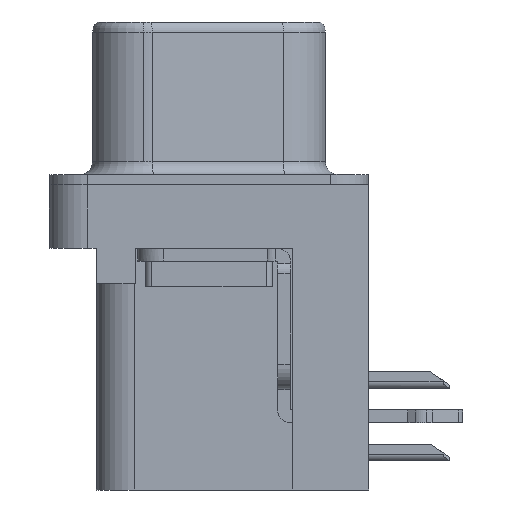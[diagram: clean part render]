
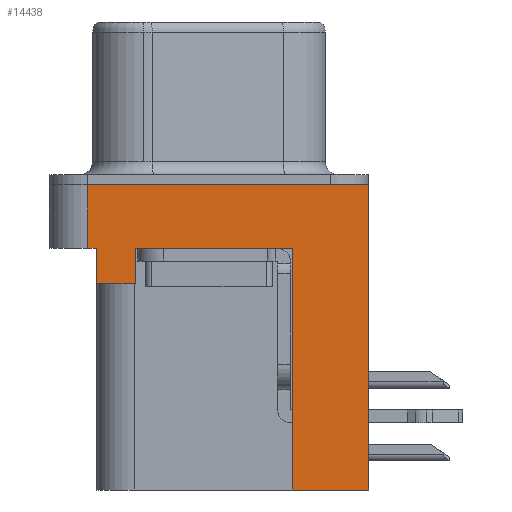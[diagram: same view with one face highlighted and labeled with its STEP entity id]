
A CAD part, left-side view. The second image highlights one B-rep face of the part: STEP entity #14438.
In plain terms, the highlighted planar face has unit normal (-1, 0, 0).
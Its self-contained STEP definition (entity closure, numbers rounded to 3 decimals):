
#424 = CARTESIAN_POINT ( 'NONE',  ( -2.91, -3.295, -12. ) ) ;
#498 = LINE ( 'NONE', #3446, #7345 ) ;
#590 = CARTESIAN_POINT ( 'NONE',  ( -2.91, -6.275, -12. ) ) ;
#839 = LINE ( 'NONE', #424, #10477 ) ;
#1128 = ORIENTED_EDGE ( 'NONE', *, *, #12893, .T. ) ;
#1135 = EDGE_CURVE ( 'NONE', #9206, #2149, #12615, .T. ) ;
#1337 = CARTESIAN_POINT ( 'NONE',  ( -2.91, -6.275, -2.5 ) ) ;
#1346 = CARTESIAN_POINT ( 'NONE',  ( -2.91, -6.275, -2.5 ) ) ;
#1500 = DIRECTION ( 'NONE',  ( 0., 1., 0. ) ) ;
#1649 = VECTOR ( 'NONE', #1500, 1000. ) ;
#1783 = VERTEX_POINT ( 'NONE', #590 ) ;
#1950 = VERTEX_POINT ( 'NONE', #9970 ) ;
#1992 = ORIENTED_EDGE ( 'NONE', *, *, #14598, .F. ) ;
#2149 = VERTEX_POINT ( 'NONE', #2398 ) ;
#2398 = CARTESIAN_POINT ( 'NONE',  ( -2.91, 4.425, -2.5 ) ) ;
#2437 = ORIENTED_EDGE ( 'NONE', *, *, #13049, .F. ) ;
#2489 = CARTESIAN_POINT ( 'NONE',  ( -2.91, 4.775, -2.5 ) ) ;
#2732 = CARTESIAN_POINT ( 'NONE',  ( -2.91, 2.895, -3.9 ) ) ;
#2968 = CARTESIAN_POINT ( 'NONE',  ( -2.91, 2.895, -3.9 ) ) ;
#3211 = CARTESIAN_POINT ( 'NONE',  ( -2.91, -6.275, 0. ) ) ;
#3323 = CARTESIAN_POINT ( 'NONE',  ( -2.91, 4.425, -3.9 ) ) ;
#3330 = DIRECTION ( 'NONE',  ( 0., -1., 0. ) ) ;
#3446 = CARTESIAN_POINT ( 'NONE',  ( -2.91, 4.425, -3.9 ) ) ;
#3449 = FACE_OUTER_BOUND ( 'NONE', #11351, .T. ) ;
#3548 = CARTESIAN_POINT ( 'NONE',  ( -2.91, 4.425, -3.9 ) ) ;
#3819 = EDGE_CURVE ( 'NONE', #14897, #7387, #4460, .T. ) ;
#4460 = LINE ( 'NONE', #3211, #14893 ) ;
#4625 = LINE ( 'NONE', #5019, #14853 ) ;
#5019 = CARTESIAN_POINT ( 'NONE',  ( -2.91, 4.775, -2.5 ) ) ;
#5184 = ORIENTED_EDGE ( 'NONE', *, *, #1135, .T. ) ;
#5431 = CARTESIAN_POINT ( 'NONE',  ( -2.91, -3.295, -12. ) ) ;
#5680 = CARTESIAN_POINT ( 'NONE',  ( -2.91, -6.275, -2.5 ) ) ;
#5758 = ORIENTED_EDGE ( 'NONE', *, *, #7703, .F. ) ;
#6206 = DIRECTION ( 'NONE',  ( 0., 1., 0. ) ) ;
#6289 = DIRECTION ( 'NONE',  ( 0., 0., 1. ) ) ;
#7345 = VECTOR ( 'NONE', #9887, 1000. ) ;
#7378 = DIRECTION ( 'NONE',  ( 0., 0., 1. ) ) ;
#7387 = VERTEX_POINT ( 'NONE', #10340 ) ;
#7674 = LINE ( 'NONE', #5431, #1649 ) ;
#7703 = EDGE_CURVE ( 'NONE', #15820, #10957, #13242, .T. ) ;
#8428 = ORIENTED_EDGE ( 'NONE', *, *, #13029, .F. ) ;
#8457 = VECTOR ( 'NONE', #10475, 1000. ) ;
#8480 = CARTESIAN_POINT ( 'NONE',  ( -2.91, -6.275, -2.5 ) ) ;
#8582 = VERTEX_POINT ( 'NONE', #11330 ) ;
#8858 = LINE ( 'NONE', #2968, #8457 ) ;
#9206 = VERTEX_POINT ( 'NONE', #2489 ) ;
#9887 = DIRECTION ( 'NONE',  ( 0., 0., 1. ) ) ;
#9970 = CARTESIAN_POINT ( 'NONE',  ( -2.91, 2.895, -2.5 ) ) ;
#10340 = CARTESIAN_POINT ( 'NONE',  ( -2.91, -6.275, 0. ) ) ;
#10442 = EDGE_CURVE ( 'NONE', #1950, #14710, #11135, .T. ) ;
#10475 = DIRECTION ( 'NONE',  ( 0., 0., 1. ) ) ;
#10477 = VECTOR ( 'NONE', #11759, 1000. ) ;
#10670 = LINE ( 'NONE', #1337, #11669 ) ;
#10957 = VERTEX_POINT ( 'NONE', #3323 ) ;
#10972 = EDGE_CURVE ( 'NONE', #10957, #2149, #498, .T. ) ;
#11135 = LINE ( 'NONE', #1346, #12361 ) ;
#11266 = CARTESIAN_POINT ( 'NONE',  ( -2.91, 4.775, 0. ) ) ;
#11330 = CARTESIAN_POINT ( 'NONE',  ( -2.91, -3.295, -12. ) ) ;
#11351 = EDGE_LOOP ( 'NONE', ( #13111, #1992, #5184, #11954, #5758, #15633, #11935, #2437, #8428, #1128 ) ) ;
#11669 = VECTOR ( 'NONE', #14252, 1000. ) ;
#11759 = DIRECTION ( 'NONE',  ( 0., 0., 1. ) ) ;
#11935 = ORIENTED_EDGE ( 'NONE', *, *, #10442, .T. ) ;
#11954 = ORIENTED_EDGE ( 'NONE', *, *, #10972, .F. ) ;
#12237 = VECTOR ( 'NONE', #6206, 1000. ) ;
#12361 = VECTOR ( 'NONE', #12961, 1000. ) ;
#12615 = LINE ( 'NONE', #5680, #14815 ) ;
#12893 = EDGE_CURVE ( 'NONE', #1783, #7387, #10670, .T. ) ;
#12905 = CARTESIAN_POINT ( 'NONE',  ( -2.91, -3.295, -2.5 ) ) ;
#12961 = DIRECTION ( 'NONE',  ( 0., -1., 0. ) ) ;
#13004 = EDGE_CURVE ( 'NONE', #15820, #1950, #8858, .T. ) ;
#13029 = EDGE_CURVE ( 'NONE', #1783, #8582, #7674, .T. ) ;
#13049 = EDGE_CURVE ( 'NONE', #8582, #14710, #839, .T. ) ;
#13111 = ORIENTED_EDGE ( 'NONE', *, *, #3819, .F. ) ;
#13242 = LINE ( 'NONE', #3548, #12237 ) ;
#13536 = AXIS2_PLACEMENT_3D ( 'NONE', #8480, #15051, #7378 ) ;
#14252 = DIRECTION ( 'NONE',  ( 0., 0., 1. ) ) ;
#14438 = ADVANCED_FACE ( 'NONE', ( #3449 ), #14996, .T. ) ;
#14598 = EDGE_CURVE ( 'NONE', #9206, #14897, #4625, .T. ) ;
#14710 = VERTEX_POINT ( 'NONE', #12905 ) ;
#14815 = VECTOR ( 'NONE', #3330, 1000. ) ;
#14853 = VECTOR ( 'NONE', #6289, 1000. ) ;
#14893 = VECTOR ( 'NONE', #16044, 1000. ) ;
#14897 = VERTEX_POINT ( 'NONE', #11266 ) ;
#14996 = PLANE ( 'NONE',  #13536 ) ;
#15051 = DIRECTION ( 'NONE',  ( -1., 0., 0. ) ) ;
#15633 = ORIENTED_EDGE ( 'NONE', *, *, #13004, .T. ) ;
#15820 = VERTEX_POINT ( 'NONE', #2732 ) ;
#16044 = DIRECTION ( 'NONE',  ( 0., -1., 0. ) ) ;
